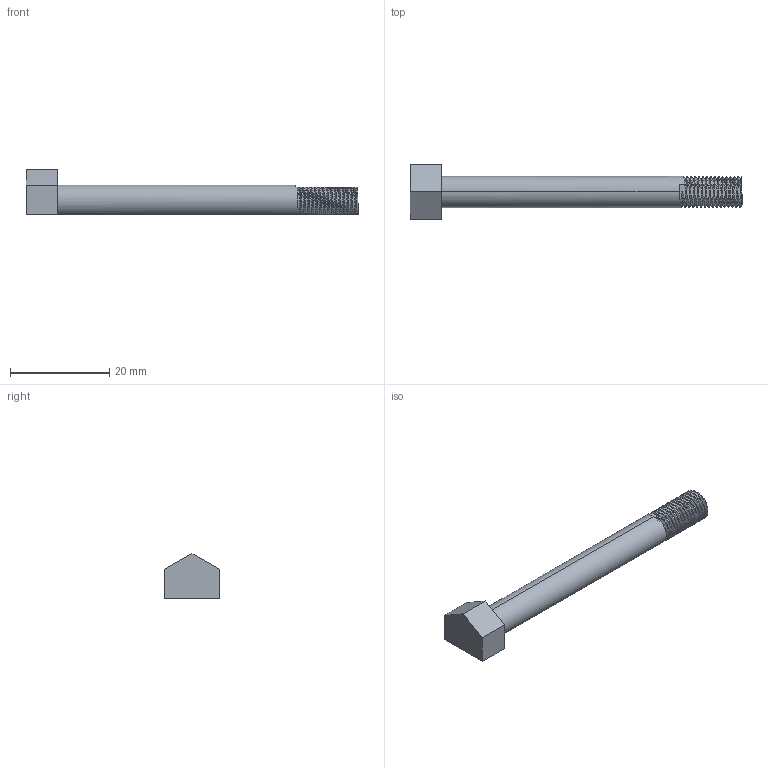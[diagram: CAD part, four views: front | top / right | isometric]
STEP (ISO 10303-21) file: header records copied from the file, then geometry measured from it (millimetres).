
FILE_DESCRIPTION (( 'STEP AP203' ), '1' );
FILE_NAME ('AF-WF-MI-PRT-005-STEP.STEP', '2020-07-21T23:27:36', ( '' ), ( '' ), 'SwSTEP 2.0', 'SolidWorks 2018', '' );
FILE_SCHEMA (( 'CONFIG_CONTROL_DESIGN' ));
Length unit declared in the file: inch
Products named in the file (1): AF-WF-MI-PRT-005-STEP
Bounding box: 67.06 x 10.92 x 9.05 mm (x, y, z)
Volume: 2332.4 mm3; surface area: 1676.1 mm2
Topology: 1 solids, 1 shells, 77 faces, 225 edges, 150 vertices
Faces by surface type: plane 41, cylinder 32, bspline 4
Entity records: 5737 total; most frequent: CARTESIAN_POINT 3953, ORIENTED_EDGE 450, DIRECTION 245, EDGE_CURVE 225, VERTEX_POINT 150, LINE 87, VECTOR 87, AXIS2_PLACEMENT_3D 79
